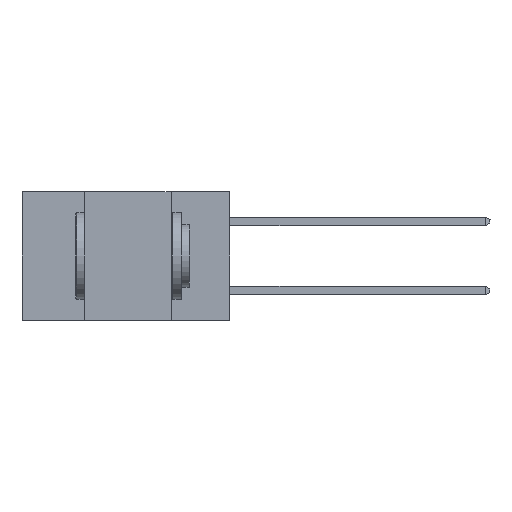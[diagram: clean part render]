
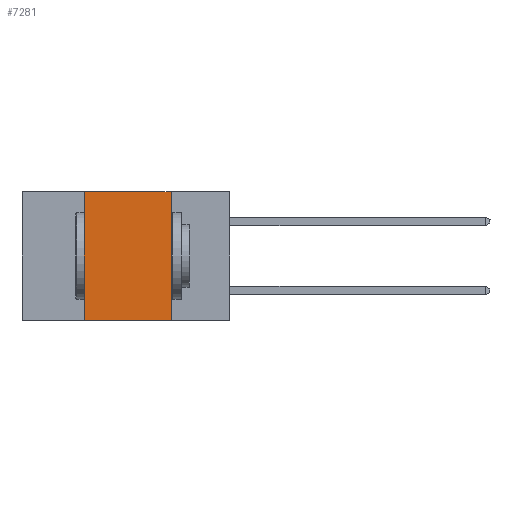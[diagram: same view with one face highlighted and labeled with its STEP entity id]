
A CAD part, left-side view. The second image highlights one B-rep face of the part: STEP entity #7281.
In plain terms, the highlighted planar face has unit normal (-1, 0, 0).
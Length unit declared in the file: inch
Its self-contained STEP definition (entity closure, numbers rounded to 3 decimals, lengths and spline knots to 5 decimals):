
#387 = VECTOR ( 'NONE', #5637, 39.37008 ) ;
#1341 = PLANE ( 'NONE',  #5689 ) ;
#1409 = ORIENTED_EDGE ( 'NONE', *, *, #9758, .F. ) ;
#1589 = VECTOR ( 'NONE', #7527, 39.37008 ) ;
#1618 = CARTESIAN_POINT ( 'NONE',  ( 0., 0.17, 0. ) ) ;
#1894 = FACE_OUTER_BOUND ( 'NONE', #5698, .T. ) ;
#2111 = VECTOR ( 'NONE', #4402, 39.37008 ) ;
#2223 = VERTEX_POINT ( 'NONE', #1618 ) ;
#2322 = DIRECTION ( 'NONE',  ( 1., 0., 0. ) ) ;
#2798 = CARTESIAN_POINT ( 'NONE',  ( 0., 0.6, -0.37 ) ) ;
#3893 = LINE ( 'NONE', #9150, #1589 ) ;
#4137 = VERTEX_POINT ( 'NONE', #9581 ) ;
#4142 = CARTESIAN_POINT ( 'NONE',  ( 0., 0.17, -0.37 ) ) ;
#4402 = DIRECTION ( 'NONE',  ( 0., -1., 0. ) ) ;
#4643 = DIRECTION ( 'NONE',  ( 0., 0., 1. ) ) ;
#4841 = ORIENTED_EDGE ( 'NONE', *, *, #8891, .F. ) ;
#5604 = CARTESIAN_POINT ( 'NONE',  ( 0., 0.6, 0. ) ) ;
#5637 = DIRECTION ( 'NONE',  ( 0., -1., 0. ) ) ;
#5689 = AXIS2_PLACEMENT_3D ( 'NONE', #8407, #2322, #10927 ) ;
#5698 = EDGE_LOOP ( 'NONE', ( #4841, #1409, #6667, #10240 ) ) ;
#6104 = VECTOR ( 'NONE', #4643, 39.37008 ) ;
#6667 = ORIENTED_EDGE ( 'NONE', *, *, #7798, .F. ) ;
#6856 = CARTESIAN_POINT ( 'NONE',  ( 0., 0.42, 0. ) ) ;
#7281 = ADVANCED_FACE ( 'NONE', ( #1894 ), #1341, .F. ) ;
#7527 = DIRECTION ( 'NONE',  ( 0., 0., -1. ) ) ;
#7798 = EDGE_CURVE ( 'NONE', #4137, #8004, #10749, .T. ) ;
#8004 = VERTEX_POINT ( 'NONE', #6856 ) ;
#8407 = CARTESIAN_POINT ( 'NONE',  ( 0., 0.6, 0. ) ) ;
#8558 = CARTESIAN_POINT ( 'NONE',  ( 0., 0.42, 0. ) ) ;
#8891 = EDGE_CURVE ( 'NONE', #2223, #8973, #3893, .T. ) ;
#8973 = VERTEX_POINT ( 'NONE', #4142 ) ;
#9150 = CARTESIAN_POINT ( 'NONE',  ( 0., 0.17, 0. ) ) ;
#9152 = EDGE_CURVE ( 'NONE', #4137, #8973, #10034, .T. ) ;
#9581 = CARTESIAN_POINT ( 'NONE',  ( 0., 0.42, -0.37 ) ) ;
#9744 = LINE ( 'NONE', #5604, #387 ) ;
#9758 = EDGE_CURVE ( 'NONE', #8004, #2223, #9744, .T. ) ;
#10034 = LINE ( 'NONE', #2798, #2111 ) ;
#10240 = ORIENTED_EDGE ( 'NONE', *, *, #9152, .T. ) ;
#10749 = LINE ( 'NONE', #8558, #6104 ) ;
#10927 = DIRECTION ( 'NONE',  ( 0., 0., -1. ) ) ;
